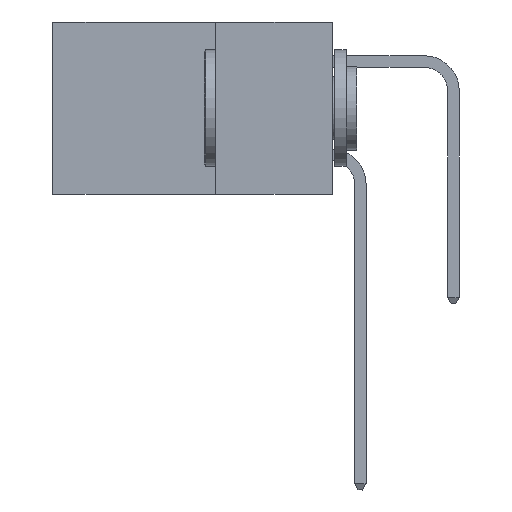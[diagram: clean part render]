
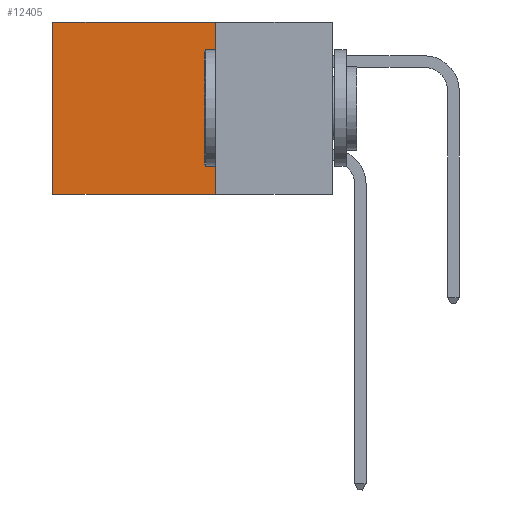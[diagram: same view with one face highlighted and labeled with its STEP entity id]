
A CAD part, left-side view. The second image highlights one B-rep face of the part: STEP entity #12405.
In plain terms, the highlighted planar face has unit normal (-1, 0, 0).
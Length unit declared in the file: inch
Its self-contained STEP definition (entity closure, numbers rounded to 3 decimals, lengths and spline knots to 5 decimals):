
#40 = ORIENTED_EDGE ( 'NONE', *, *, #3581, .T. ) ;
#375 = CARTESIAN_POINT ( 'NONE',  ( 0.298, 0.25, 0. ) ) ;
#558 = DIRECTION ( 'NONE',  ( 0., 1., 0. ) ) ;
#1476 = DIRECTION ( 'NONE',  ( 0., 1., 0. ) ) ;
#2843 = EDGE_LOOP ( 'NONE', ( #12853, #9550, #12753, #40 ) ) ;
#2934 = VERTEX_POINT ( 'NONE', #10948 ) ;
#2971 = PLANE ( 'NONE',  #4119 ) ;
#3015 = EDGE_CURVE ( 'NONE', #13745, #4021, #12398, .T. ) ;
#3581 = EDGE_CURVE ( 'NONE', #13745, #12811, #7484, .T. ) ;
#4021 = VERTEX_POINT ( 'NONE', #8524 ) ;
#4104 = VECTOR ( 'NONE', #558, 39.37008 ) ;
#4119 = AXIS2_PLACEMENT_3D ( 'NONE', #375, #11830, #4297 ) ;
#4297 = DIRECTION ( 'NONE',  ( 0., 0., -1. ) ) ;
#4737 = FACE_OUTER_BOUND ( 'NONE', #2843, .T. ) ;
#6232 = CARTESIAN_POINT ( 'NONE',  ( 0.298, 0.6, 0. ) ) ;
#6666 = CARTESIAN_POINT ( 'NONE',  ( 0.298, 0.25, -0.37 ) ) ;
#7409 = EDGE_CURVE ( 'NONE', #12811, #2934, #14956, .T. ) ;
#7484 = LINE ( 'NONE', #13504, #4104 ) ;
#7505 = CARTESIAN_POINT ( 'NONE',  ( 0.298, 0.25, 0. ) ) ;
#7599 = CARTESIAN_POINT ( 'NONE',  ( 0.298, 0.25, 0. ) ) ;
#8318 = VECTOR ( 'NONE', #10957, 39.37008 ) ;
#8370 = CARTESIAN_POINT ( 'NONE',  ( 0.298, 0.6, 0. ) ) ;
#8524 = CARTESIAN_POINT ( 'NONE',  ( 0.298, 0.25, -0.37 ) ) ;
#9550 = ORIENTED_EDGE ( 'NONE', *, *, #11680, .F. ) ;
#10451 = VECTOR ( 'NONE', #1476, 39.37008 ) ;
#10948 = CARTESIAN_POINT ( 'NONE',  ( 0.298, 0.6, -0.37 ) ) ;
#10957 = DIRECTION ( 'NONE',  ( 0., 0., -1. ) ) ;
#11680 = EDGE_CURVE ( 'NONE', #4021, #2934, #13787, .T. ) ;
#11830 = DIRECTION ( 'NONE',  ( 1., 0., 0. ) ) ;
#12398 = LINE ( 'NONE', #7505, #14905 ) ;
#12405 = ADVANCED_FACE ( 'NONE', ( #4737 ), #2971, .F. ) ;
#12632 = DIRECTION ( 'NONE',  ( 0., 0., -1. ) ) ;
#12753 = ORIENTED_EDGE ( 'NONE', *, *, #3015, .F. ) ;
#12811 = VERTEX_POINT ( 'NONE', #6232 ) ;
#12853 = ORIENTED_EDGE ( 'NONE', *, *, #7409, .T. ) ;
#13504 = CARTESIAN_POINT ( 'NONE',  ( 0.298, 0.25, 0. ) ) ;
#13745 = VERTEX_POINT ( 'NONE', #7599 ) ;
#13787 = LINE ( 'NONE', #6666, #10451 ) ;
#14905 = VECTOR ( 'NONE', #12632, 39.37008 ) ;
#14956 = LINE ( 'NONE', #8370, #8318 ) ;
